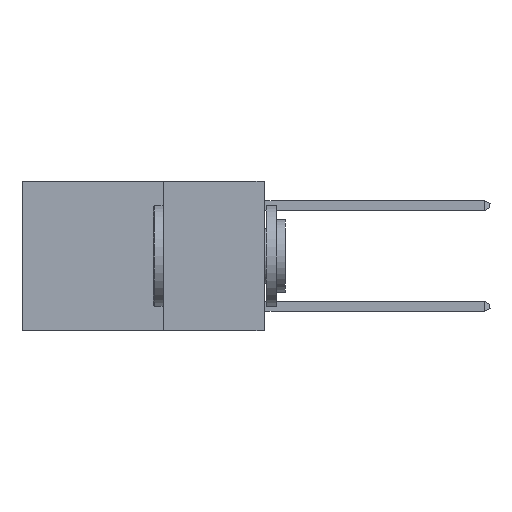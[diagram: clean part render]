
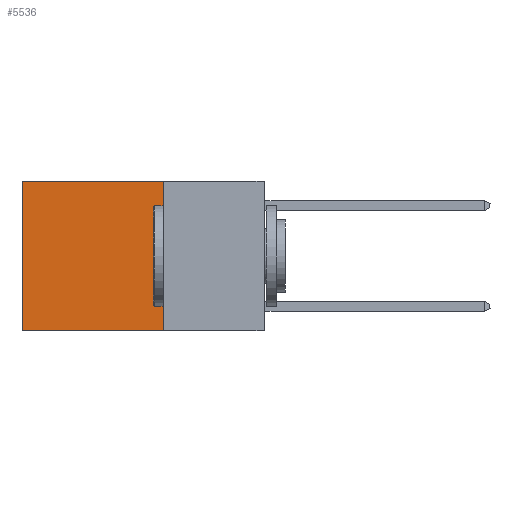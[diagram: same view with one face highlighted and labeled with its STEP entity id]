
A CAD part, left-side view. The second image highlights one B-rep face of the part: STEP entity #5536.
In plain terms, the highlighted planar face has unit normal (-1, 0, 0).
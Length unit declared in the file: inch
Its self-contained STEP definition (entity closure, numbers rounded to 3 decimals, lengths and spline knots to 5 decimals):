
#737 = DIRECTION ( 'NONE',  ( 0., 0., -1. ) ) ;
#834 = CARTESIAN_POINT ( 'NONE',  ( 0.2625, 0.25, 0. ) ) ;
#1576 = CARTESIAN_POINT ( 'NONE',  ( 0.2625, 0.25, -0.37 ) ) ;
#2776 = DIRECTION ( 'NONE',  ( 0., 1., 0. ) ) ;
#3388 = EDGE_CURVE ( 'NONE', #19495, #15803, #15716, .T. ) ;
#3705 = ORIENTED_EDGE ( 'NONE', *, *, #15025, .F. ) ;
#3750 = DIRECTION ( 'NONE',  ( 0., 1., 0. ) ) ;
#3822 = FACE_OUTER_BOUND ( 'NONE', #14456, .T. ) ;
#3958 = CARTESIAN_POINT ( 'NONE',  ( 0.2625, 0.25, 0. ) ) ;
#4182 = VECTOR ( 'NONE', #3750, 39.37008 ) ;
#4542 = VERTEX_POINT ( 'NONE', #10621 ) ;
#4546 = LINE ( 'NONE', #10605, #14376 ) ;
#5098 = LINE ( 'NONE', #10852, #6774 ) ;
#5536 = ADVANCED_FACE ( 'NONE', ( #3822 ), #11184, .F. ) ;
#6774 = VECTOR ( 'NONE', #10966, 39.37008 ) ;
#10605 = CARTESIAN_POINT ( 'NONE',  ( 0.2625, 0.6, 0. ) ) ;
#10621 = CARTESIAN_POINT ( 'NONE',  ( 0.2625, 0.25, -0.37 ) ) ;
#10643 = EDGE_CURVE ( 'NONE', #4542, #12218, #16436, .T. ) ;
#10852 = CARTESIAN_POINT ( 'NONE',  ( 0.2625, 0.25, 0. ) ) ;
#10966 = DIRECTION ( 'NONE',  ( 0., 0., -1. ) ) ;
#11111 = CARTESIAN_POINT ( 'NONE',  ( 0.2625, 0.6, 0. ) ) ;
#11184 = PLANE ( 'NONE',  #17329 ) ;
#11246 = CARTESIAN_POINT ( 'NONE',  ( 0.2625, 0.6, -0.37 ) ) ;
#11432 = ORIENTED_EDGE ( 'NONE', *, *, #10643, .F. ) ;
#12045 = ORIENTED_EDGE ( 'NONE', *, *, #18658, .T. ) ;
#12218 = VERTEX_POINT ( 'NONE', #11246 ) ;
#14270 = ORIENTED_EDGE ( 'NONE', *, *, #3388, .T. ) ;
#14376 = VECTOR ( 'NONE', #16719, 39.37008 ) ;
#14456 = EDGE_LOOP ( 'NONE', ( #12045, #11432, #3705, #14270 ) ) ;
#14576 = CARTESIAN_POINT ( 'NONE',  ( 0.2625, 0.25, 0. ) ) ;
#15025 = EDGE_CURVE ( 'NONE', #19495, #4542, #5098, .T. ) ;
#15221 = VECTOR ( 'NONE', #2776, 39.37008 ) ;
#15716 = LINE ( 'NONE', #3958, #4182 ) ;
#15803 = VERTEX_POINT ( 'NONE', #11111 ) ;
#15891 = DIRECTION ( 'NONE',  ( 1., 0., 0. ) ) ;
#16436 = LINE ( 'NONE', #1576, #15221 ) ;
#16719 = DIRECTION ( 'NONE',  ( 0., 0., -1. ) ) ;
#17329 = AXIS2_PLACEMENT_3D ( 'NONE', #14576, #15891, #737 ) ;
#18658 = EDGE_CURVE ( 'NONE', #15803, #12218, #4546, .T. ) ;
#19495 = VERTEX_POINT ( 'NONE', #834 ) ;
